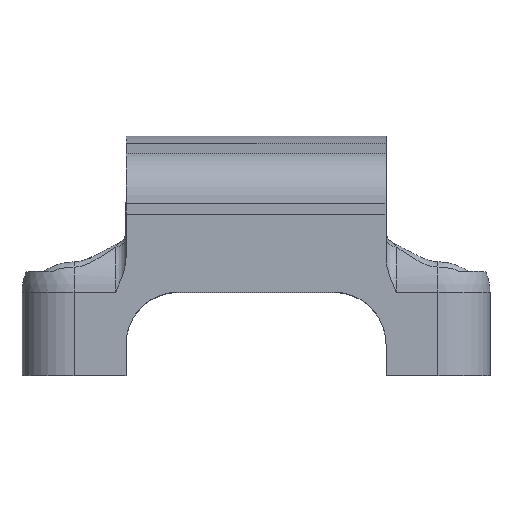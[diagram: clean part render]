
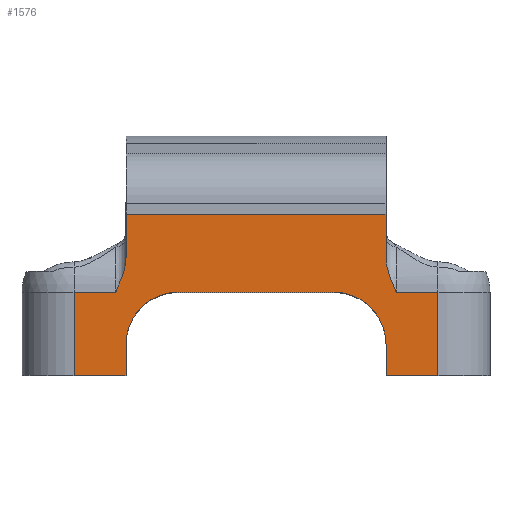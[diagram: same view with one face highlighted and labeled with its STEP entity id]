
A CAD part, top view. The second image highlights one B-rep face of the part: STEP entity #1576.
In plain terms, the highlighted planar face has unit normal (0, 0, 1).
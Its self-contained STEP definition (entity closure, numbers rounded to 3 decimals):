
#65 = LINE ( 'NONE', #1897, #66 ) ;
#66 = VECTOR ( 'NONE', #1886, 1000. ) ;
#84 = VECTOR ( 'NONE', #1348, 1000. ) ;
#85 = CARTESIAN_POINT ( 'NONE',  ( -6.25, -6.5, 7.5 ) ) ;
#106 = CARTESIAN_POINT ( 'NONE',  ( 6.25, -2.5, 7.5 ) ) ;
#237 = CARTESIAN_POINT ( 'NONE',  ( 8.75, -2.5, 7.5 ) ) ;
#252 = DIRECTION ( 'NONE',  ( 1., 0., 0. ) ) ;
#304 = CARTESIAN_POINT ( 'NONE',  ( 6.329, -1.415, 7.5 ) ) ;
#341 = DIRECTION ( 'NONE',  ( 0., 1., 0. ) ) ;
#347 = CARTESIAN_POINT ( 'NONE',  ( -8.75, -2.5, 7.5 ) ) ;
#357 = ORIENTED_EDGE ( 'NONE', *, *, #1742, .T. ) ;
#362 = ORIENTED_EDGE ( 'NONE', *, *, #2645, .T. ) ;
#373 = CARTESIAN_POINT ( 'NONE',  ( -6.25, 0., 7.5 ) ) ;
#374 = EDGE_CURVE ( 'NONE', #1562, #1209, #65, .T. ) ;
#380 = CARTESIAN_POINT ( 'NONE',  ( -6.25, 0., 7.5 ) ) ;
#393 = ORIENTED_EDGE ( 'NONE', *, *, #2415, .F. ) ;
#417 = ORIENTED_EDGE ( 'NONE', *, *, #1971, .T. ) ;
#424 = B_SPLINE_CURVE_WITH_KNOTS ( 'NONE', 3,
 ( #1550, #1344, #1414, #2074, #304, #1229, #1330, #698 ),
 .UNSPECIFIED., .F., .F.,
 ( 4, 2, 2, 4 ),
 ( 0., 0.001, 0.001, 0.002 ),
 .UNSPECIFIED. ) ;
#431 = ORIENTED_EDGE ( 'NONE', *, *, #826, .T. ) ;
#445 = CARTESIAN_POINT ( 'NONE',  ( 3.75, -2.5, 7.5 ) ) ;
#459 = CARTESIAN_POINT ( 'NONE',  ( -6.75, -2.5, 7.5 ) ) ;
#460 = ORIENTED_EDGE ( 'NONE', *, *, #531, .F. ) ;
#482 = ORIENTED_EDGE ( 'NONE', *, *, #1136, .T. ) ;
#531 = EDGE_CURVE ( 'NONE', #1209, #603, #2305, .T. ) ;
#549 = VERTEX_POINT ( 'NONE', #1062 ) ;
#603 = VERTEX_POINT ( 'NONE', #930 ) ;
#615 = VECTOR ( 'NONE', #2511, 1000. ) ;
#629 = ORIENTED_EDGE ( 'NONE', *, *, #1014, .T. ) ;
#630 = LINE ( 'NONE', #2603, #615 ) ;
#636 = VERTEX_POINT ( 'NONE', #804 ) ;
#641 = ORIENTED_EDGE ( 'NONE', *, *, #2536, .T. ) ;
#649 = CARTESIAN_POINT ( 'NONE',  ( -6.512, -1.969, 7.5 ) ) ;
#652 = EDGE_CURVE ( 'NONE', #1382, #603, #2513, .T. ) ;
#665 = ORIENTED_EDGE ( 'NONE', *, *, #2118, .T. ) ;
#675 = ORIENTED_EDGE ( 'NONE', *, *, #1159, .T. ) ;
#698 = CARTESIAN_POINT ( 'NONE',  ( 6.25, -0.842, 7.5 ) ) ;
#702 = ORIENTED_EDGE ( 'NONE', *, *, #652, .T. ) ;
#709 = ORIENTED_EDGE ( 'NONE', *, *, #374, .F. ) ;
#744 = DIRECTION ( 'NONE',  ( 1., 0., 0. ) ) ;
#748 = DIRECTION ( 'NONE',  ( 0., 0., -1. ) ) ;
#755 = CARTESIAN_POINT ( 'NONE',  ( 3.75, -5., 7.5 ) ) ;
#797 = EDGE_LOOP ( 'NONE', ( #357, #629, #362, #641, #393, #1093, #665, #417, #1112, #1851, #675, #431, #702, #460, #709, #482 ) ) ;
#804 = CARTESIAN_POINT ( 'NONE',  ( 6.25, -0.842, 7.5 ) ) ;
#826 = EDGE_CURVE ( 'NONE', #2011, #1382, #2077, .T. ) ;
#845 = AXIS2_PLACEMENT_3D ( 'NONE', #2557, #1096, #2368 ) ;
#851 = CARTESIAN_POINT ( 'NONE',  ( -6.329, -1.416, 7.5 ) ) ;
#930 = CARTESIAN_POINT ( 'NONE',  ( 6.25, -5., 7.5 ) ) ;
#962 = CARTESIAN_POINT ( 'NONE',  ( 6.25, -6.5, 7.5 ) ) ;
#963 = VECTOR ( 'NONE', #1298, 1000. ) ;
#965 = LINE ( 'NONE', #1078, #963 ) ;
#1012 = VERTEX_POINT ( 'NONE', #85 ) ;
#1014 = EDGE_CURVE ( 'NONE', #1188, #636, #424, .T. ) ;
#1058 = CARTESIAN_POINT ( 'NONE',  ( -6.25, -0.989, 7.5 ) ) ;
#1062 = CARTESIAN_POINT ( 'NONE',  ( -6.75, -2.5, 7.5 ) ) ;
#1078 = CARTESIAN_POINT ( 'NONE',  ( 0., 1.25, 7.5 ) ) ;
#1093 = ORIENTED_EDGE ( 'NONE', *, *, #2268, .T. ) ;
#1096 = DIRECTION ( 'NONE',  ( 0., 0., 1. ) ) ;
#1109 = CARTESIAN_POINT ( 'NONE',  ( -3.75, -2.5, 7.5 ) ) ;
#1112 = ORIENTED_EDGE ( 'NONE', *, *, #1645, .T. ) ;
#1136 = EDGE_CURVE ( 'NONE', #1562, #2274, #1517, .T. ) ;
#1159 = EDGE_CURVE ( 'NONE', #1931, #2011, #1275, .T. ) ;
#1180 = VECTOR ( 'NONE', #2041, 1000. ) ;
#1184 = LINE ( 'NONE', #373, #1180 ) ;
#1188 = VERTEX_POINT ( 'NONE', #1205 ) ;
#1205 = CARTESIAN_POINT ( 'NONE',  ( 6.75, -2.5, 7.5 ) ) ;
#1209 = VERTEX_POINT ( 'NONE', #962 ) ;
#1229 = CARTESIAN_POINT ( 'NONE',  ( 6.269, -1.132, 7.5 ) ) ;
#1240 = AXIS2_PLACEMENT_3D ( 'NONE', #2236, #2230, #2206 ) ;
#1275 = CIRCLE ( 'NONE', #1240, 2.5 ) ;
#1298 = DIRECTION ( 'NONE',  ( -1., 0., 0. ) ) ;
#1315 = PLANE ( 'NONE',  #845 ) ;
#1330 = CARTESIAN_POINT ( 'NONE',  ( 6.25, -0.989, 7.5 ) ) ;
#1344 = CARTESIAN_POINT ( 'NONE',  ( 6.631, -2.234, 7.5 ) ) ;
#1348 = DIRECTION ( 'NONE',  ( 0., 1., 0. ) ) ;
#1373 = CARTESIAN_POINT ( 'NONE',  ( 6.25, 0., 7.5 ) ) ;
#1382 = VERTEX_POINT ( 'NONE', #445 ) ;
#1392 = EDGE_CURVE ( 'NONE', #1012, #1931, #2468, .T. ) ;
#1414 = CARTESIAN_POINT ( 'NONE',  ( 6.512, -1.969, 7.5 ) ) ;
#1486 = VERTEX_POINT ( 'NONE', #1665 ) ;
#1517 = LINE ( 'NONE', #2601, #1712 ) ;
#1550 = CARTESIAN_POINT ( 'NONE',  ( 6.75, -2.5, 7.5 ) ) ;
#1562 = VERTEX_POINT ( 'NONE', #2521 ) ;
#1568 = VECTOR ( 'NONE', #1719, 1000. ) ;
#1576 = ADVANCED_FACE ( 'NONE', ( #2410 ), #1315, .T. ) ;
#1596 = CARTESIAN_POINT ( 'NONE',  ( -6.25, -0.842, 7.5 ) ) ;
#1620 = CARTESIAN_POINT ( 'NONE',  ( -6.25, -5., 7.5 ) ) ;
#1629 = LINE ( 'NONE', #2356, #1568 ) ;
#1645 = EDGE_CURVE ( 'NONE', #1663, #1012, #2655, .T. ) ;
#1661 = DIRECTION ( 'NONE',  ( 0., -1., 0. ) ) ;
#1663 = VERTEX_POINT ( 'NONE', #1715 ) ;
#1665 = CARTESIAN_POINT ( 'NONE',  ( -6.25, -0.842, 7.5 ) ) ;
#1712 = VECTOR ( 'NONE', #2652, 1000. ) ;
#1715 = CARTESIAN_POINT ( 'NONE',  ( -8.75, -6.5, 7.5 ) ) ;
#1717 = CARTESIAN_POINT ( 'NONE',  ( 0., -2.5, 7.5 ) ) ;
#1719 = DIRECTION ( 'NONE',  ( -1., 0., 0. ) ) ;
#1742 = EDGE_CURVE ( 'NONE', #2274, #1188, #2247, .T. ) ;
#1851 = ORIENTED_EDGE ( 'NONE', *, *, #1392, .T. ) ;
#1852 = VECTOR ( 'NONE', #1661, 1000. ) ;
#1857 = LINE ( 'NONE', #2263, #1852 ) ;
#1877 = AXIS2_PLACEMENT_3D ( 'NONE', #755, #748, #744 ) ;
#1883 = VECTOR ( 'NONE', #252, 1000. ) ;
#1886 = DIRECTION ( 'NONE',  ( -1., 0., 0. ) ) ;
#1897 = CARTESIAN_POINT ( 'NONE',  ( 0., -6.5, 7.5 ) ) ;
#1912 = CARTESIAN_POINT ( 'NONE',  ( -6.632, -2.236, 7.5 ) ) ;
#1931 = VERTEX_POINT ( 'NONE', #1620 ) ;
#1971 = EDGE_CURVE ( 'NONE', #2266, #1663, #1857, .T. ) ;
#2011 = VERTEX_POINT ( 'NONE', #1109 ) ;
#2041 = DIRECTION ( 'NONE',  ( 0., 1., 0. ) ) ;
#2074 = CARTESIAN_POINT ( 'NONE',  ( 6.37, -1.556, 7.5 ) ) ;
#2077 = LINE ( 'NONE', #1717, #1883 ) ;
#2116 = VECTOR ( 'NONE', #2583, 1000. ) ;
#2118 = EDGE_CURVE ( 'NONE', #549, #2266, #1629, .T. ) ;
#2124 = CARTESIAN_POINT ( 'NONE',  ( -6.37, -1.556, 7.5 ) ) ;
#2140 = CARTESIAN_POINT ( 'NONE',  ( 0., -6.5, 7.5 ) ) ;
#2206 = DIRECTION ( 'NONE',  ( 1., 0., 0. ) ) ;
#2216 = VECTOR ( 'NONE', #2351, 1000. ) ;
#2230 = DIRECTION ( 'NONE',  ( 0., 0., -1. ) ) ;
#2236 = CARTESIAN_POINT ( 'NONE',  ( -3.75, -5., 7.5 ) ) ;
#2247 = LINE ( 'NONE', #106, #2116 ) ;
#2263 = CARTESIAN_POINT ( 'NONE',  ( -8.75, 0., 7.5 ) ) ;
#2266 = VERTEX_POINT ( 'NONE', #347 ) ;
#2268 = EDGE_CURVE ( 'NONE', #1486, #549, #2427, .T. ) ;
#2274 = VERTEX_POINT ( 'NONE', #237 ) ;
#2305 = LINE ( 'NONE', #1373, #84 ) ;
#2329 = CARTESIAN_POINT ( 'NONE',  ( -6.269, -1.132, 7.5 ) ) ;
#2351 = DIRECTION ( 'NONE',  ( 1., 0., 0. ) ) ;
#2356 = CARTESIAN_POINT ( 'NONE',  ( 0., -2.5, 7.5 ) ) ;
#2368 = DIRECTION ( 'NONE',  ( 1., 0., 0. ) ) ;
#2410 = FACE_OUTER_BOUND ( 'NONE', #797, .T. ) ;
#2415 = EDGE_CURVE ( 'NONE', #1486, #2439, #1184, .T. ) ;
#2420 = VERTEX_POINT ( 'NONE', #2625 ) ;
#2427 = B_SPLINE_CURVE_WITH_KNOTS ( 'NONE', 3,
 ( #1596, #1058, #2329, #851, #2124, #649, #1912, #459 ),
 .UNSPECIFIED., .F., .F.,
 ( 4, 2, 2, 4 ),
 ( 0., 0., 0.001, 0.002 ),
 .UNSPECIFIED. ) ;
#2439 = VERTEX_POINT ( 'NONE', #2448 ) ;
#2448 = CARTESIAN_POINT ( 'NONE',  ( -6.25, 1.25, 7.5 ) ) ;
#2464 = VECTOR ( 'NONE', #341, 1000. ) ;
#2468 = LINE ( 'NONE', #380, #2464 ) ;
#2511 = DIRECTION ( 'NONE',  ( 0., 1., 0. ) ) ;
#2513 = CIRCLE ( 'NONE', #1877, 2.5 ) ;
#2521 = CARTESIAN_POINT ( 'NONE',  ( 8.75, -6.5, 7.5 ) ) ;
#2536 = EDGE_CURVE ( 'NONE', #2420, #2439, #965, .T. ) ;
#2557 = CARTESIAN_POINT ( 'NONE',  ( 0., 0., 7.5 ) ) ;
#2583 = DIRECTION ( 'NONE',  ( -1., 0., 0. ) ) ;
#2601 = CARTESIAN_POINT ( 'NONE',  ( 8.75, -2.5, 7.5 ) ) ;
#2603 = CARTESIAN_POINT ( 'NONE',  ( 6.25, 0., 7.5 ) ) ;
#2625 = CARTESIAN_POINT ( 'NONE',  ( 6.25, 1.25, 7.5 ) ) ;
#2645 = EDGE_CURVE ( 'NONE', #636, #2420, #630, .T. ) ;
#2652 = DIRECTION ( 'NONE',  ( 0., 1., 0. ) ) ;
#2655 = LINE ( 'NONE', #2140, #2216 ) ;
